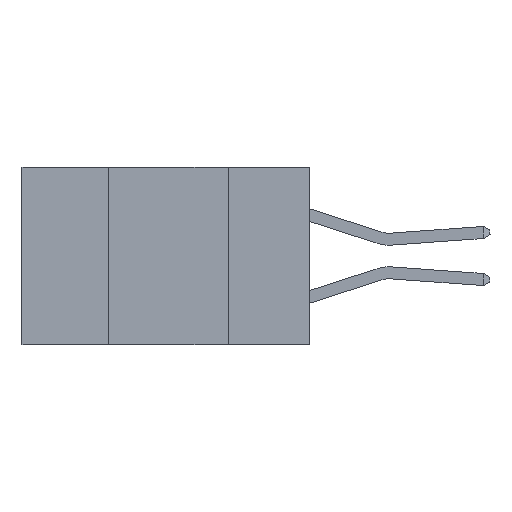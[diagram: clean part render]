
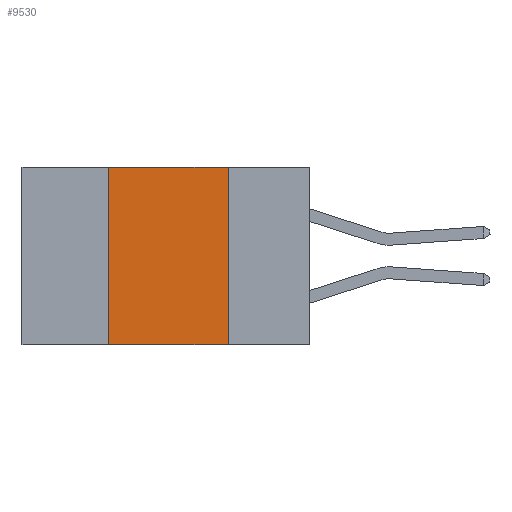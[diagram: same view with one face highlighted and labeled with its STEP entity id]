
A CAD part, left-side view. The second image highlights one B-rep face of the part: STEP entity #9530.
In plain terms, the highlighted planar face has unit normal (-1, 0, 0).
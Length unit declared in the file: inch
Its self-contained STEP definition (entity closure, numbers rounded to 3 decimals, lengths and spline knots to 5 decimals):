
#174 = ORIENTED_EDGE ( 'NONE', *, *, #17222, .F. ) ;
#894 = CARTESIAN_POINT ( 'NONE',  ( 0., 0.6, 0. ) ) ;
#1134 = VECTOR ( 'NONE', #22785, 39.37008 ) ;
#2379 = ORIENTED_EDGE ( 'NONE', *, *, #3679, .F. ) ;
#3047 = VERTEX_POINT ( 'NONE', #11979 ) ;
#3679 = EDGE_CURVE ( 'NONE', #12349, #10208, #5665, .T. ) ;
#3830 = DIRECTION ( 'NONE',  ( 0., 0., -1. ) ) ;
#4387 = DIRECTION ( 'NONE',  ( 1., 0., 0. ) ) ;
#5665 = LINE ( 'NONE', #17026, #11204 ) ;
#5828 = CARTESIAN_POINT ( 'NONE',  ( 0., 0.6, -0.37 ) ) ;
#6801 = CARTESIAN_POINT ( 'NONE',  ( 0., 0.42, 0. ) ) ;
#7115 = CARTESIAN_POINT ( 'NONE',  ( 0., 0.17, 0. ) ) ;
#8920 = ORIENTED_EDGE ( 'NONE', *, *, #19958, .F. ) ;
#9530 = ADVANCED_FACE ( 'NONE', ( #14600 ), #15021, .F. ) ;
#9906 = CARTESIAN_POINT ( 'NONE',  ( 0., 0.42, 0. ) ) ;
#10208 = VERTEX_POINT ( 'NONE', #7115 ) ;
#11204 = VECTOR ( 'NONE', #11756, 39.37008 ) ;
#11756 = DIRECTION ( 'NONE',  ( 0., -1., 0. ) ) ;
#11979 = CARTESIAN_POINT ( 'NONE',  ( 0., 0.42, -0.37 ) ) ;
#12349 = VERTEX_POINT ( 'NONE', #9906 ) ;
#12396 = VERTEX_POINT ( 'NONE', #16798 ) ;
#12411 = LINE ( 'NONE', #5828, #17697 ) ;
#12764 = LINE ( 'NONE', #16332, #21647 ) ;
#12975 = EDGE_CURVE ( 'NONE', #3047, #12396, #12411, .T. ) ;
#13840 = AXIS2_PLACEMENT_3D ( 'NONE', #894, #4387, #16795 ) ;
#14600 = FACE_OUTER_BOUND ( 'NONE', #18108, .T. ) ;
#15021 = PLANE ( 'NONE',  #13840 ) ;
#16332 = CARTESIAN_POINT ( 'NONE',  ( 0., 0.17, 0. ) ) ;
#16795 = DIRECTION ( 'NONE',  ( 0., 0., -1. ) ) ;
#16798 = CARTESIAN_POINT ( 'NONE',  ( 0., 0.17, -0.37 ) ) ;
#17026 = CARTESIAN_POINT ( 'NONE',  ( 0., 0.6, 0. ) ) ;
#17222 = EDGE_CURVE ( 'NONE', #10208, #12396, #12764, .T. ) ;
#17680 = ORIENTED_EDGE ( 'NONE', *, *, #12975, .T. ) ;
#17697 = VECTOR ( 'NONE', #20887, 39.37008 ) ;
#18108 = EDGE_LOOP ( 'NONE', ( #174, #2379, #8920, #17680 ) ) ;
#19958 = EDGE_CURVE ( 'NONE', #3047, #12349, #20605, .T. ) ;
#20605 = LINE ( 'NONE', #6801, #1134 ) ;
#20887 = DIRECTION ( 'NONE',  ( 0., -1., 0. ) ) ;
#21647 = VECTOR ( 'NONE', #3830, 39.37008 ) ;
#22785 = DIRECTION ( 'NONE',  ( 0., 0., 1. ) ) ;
